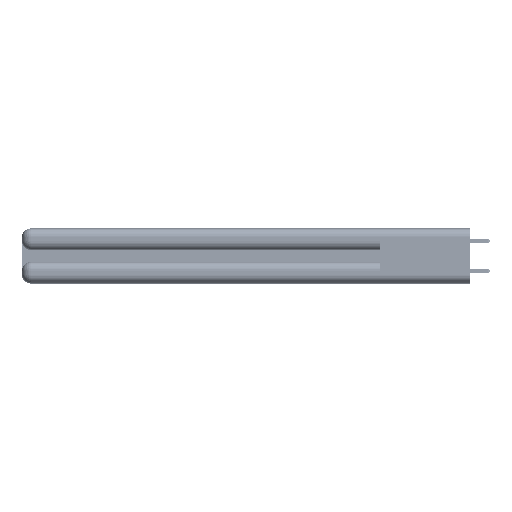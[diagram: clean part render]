
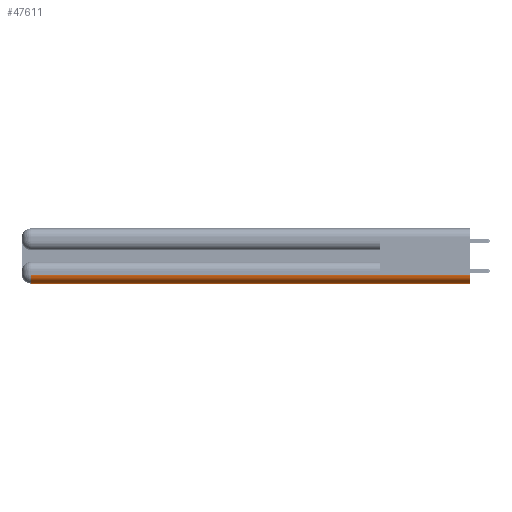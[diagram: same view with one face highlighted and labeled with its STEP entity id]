
A CAD part, left-side view. The second image highlights one B-rep face of the part: STEP entity #47611.
In plain terms, the highlighted cylindrical face has radius 1.524 mm (diameter 3.048 mm), a partial arc.
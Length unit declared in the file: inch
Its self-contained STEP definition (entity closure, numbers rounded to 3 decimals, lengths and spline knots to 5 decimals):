
#77 = EDGE_CURVE ( 'NONE', #20678, #50744, #44604, .T. ) ;
#2769 = CIRCLE ( 'NONE', #5923, 0.06 ) ;
#4735 = ORIENTED_EDGE ( 'NONE', *, *, #48548, .F. ) ;
#5560 = DIRECTION ( 'NONE',  ( 0., 0., 1. ) ) ;
#5669 = DIRECTION ( 'NONE',  ( 0., 0., 1. ) ) ;
#5676 = DIRECTION ( 'NONE',  ( 0., 1., 0. ) ) ;
#5923 = AXIS2_PLACEMENT_3D ( 'NONE', #16038, #33766, #16433 ) ;
#6323 = DIRECTION ( 'NONE',  ( 0., 1., 0. ) ) ;
#7637 = CARTESIAN_POINT ( 'NONE',  ( 0.06, 2.94, 0. ) ) ;
#11917 = VECTOR ( 'NONE', #5676, 39.37008 ) ;
#14319 = VERTEX_POINT ( 'NONE', #7637 ) ;
#16038 = CARTESIAN_POINT ( 'NONE',  ( 0.06, 2.94, 0.06 ) ) ;
#16433 = DIRECTION ( 'NONE',  ( 0., 0., 1. ) ) ;
#18652 = CARTESIAN_POINT ( 'NONE',  ( 0., 0., 0.06 ) ) ;
#20678 = VERTEX_POINT ( 'NONE', #18652 ) ;
#21654 = CYLINDRICAL_SURFACE ( 'NONE', #30228, 0.06 ) ;
#23565 = CARTESIAN_POINT ( 'NONE',  ( 0.06, 3., 0. ) ) ;
#26799 = ORIENTED_EDGE ( 'NONE', *, *, #77, .F. ) ;
#28006 = CARTESIAN_POINT ( 'NONE',  ( 0.06, 0., 0.06 ) ) ;
#28198 = DIRECTION ( 'NONE',  ( 0., -1., 0. ) ) ;
#30228 = AXIS2_PLACEMENT_3D ( 'NONE', #54449, #6323, #5560 ) ;
#31983 = FACE_OUTER_BOUND ( 'NONE', #33306, .T. ) ;
#33306 = EDGE_LOOP ( 'NONE', ( #26799, #45294, #51351, #4735 ) ) ;
#33766 = DIRECTION ( 'NONE',  ( 0., 1., 0. ) ) ;
#35337 = LINE ( 'NONE', #23565, #11917 ) ;
#44516 = LINE ( 'NONE', #49160, #54839 ) ;
#44604 = CIRCLE ( 'NONE', #47392, 0.06 ) ;
#44716 = DIRECTION ( 'NONE',  ( 0., -1., 0. ) ) ;
#45294 = ORIENTED_EDGE ( 'NONE', *, *, #56786, .F. ) ;
#46412 = VERTEX_POINT ( 'NONE', #52161 ) ;
#47392 = AXIS2_PLACEMENT_3D ( 'NONE', #28006, #28198, #5669 ) ;
#47611 = ADVANCED_FACE ( 'NONE', ( #31983 ), #21654, .T. ) ;
#48548 = EDGE_CURVE ( 'NONE', #50744, #14319, #35337, .T. ) ;
#49160 = CARTESIAN_POINT ( 'NONE',  ( 0., 0., 0.06 ) ) ;
#50744 = VERTEX_POINT ( 'NONE', #51852 ) ;
#50787 = EDGE_CURVE ( 'NONE', #14319, #46412, #2769, .T. ) ;
#51351 = ORIENTED_EDGE ( 'NONE', *, *, #50787, .F. ) ;
#51852 = CARTESIAN_POINT ( 'NONE',  ( 0.06, 0., 0. ) ) ;
#52161 = CARTESIAN_POINT ( 'NONE',  ( 0., 2.94, 0.06 ) ) ;
#54449 = CARTESIAN_POINT ( 'NONE',  ( 0.06, 0., 0.06 ) ) ;
#54839 = VECTOR ( 'NONE', #44716, 39.37008 ) ;
#56786 = EDGE_CURVE ( 'NONE', #46412, #20678, #44516, .T. ) ;
